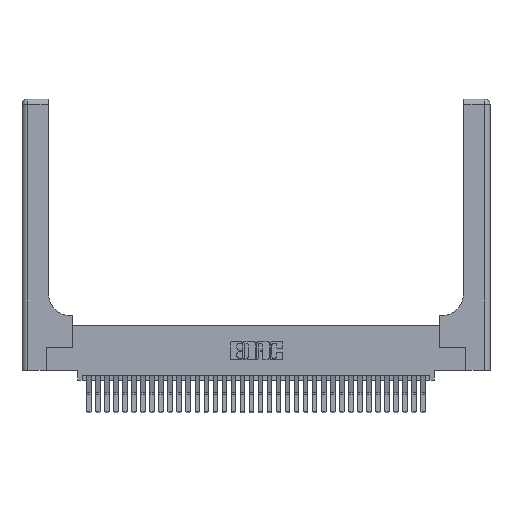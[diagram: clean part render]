
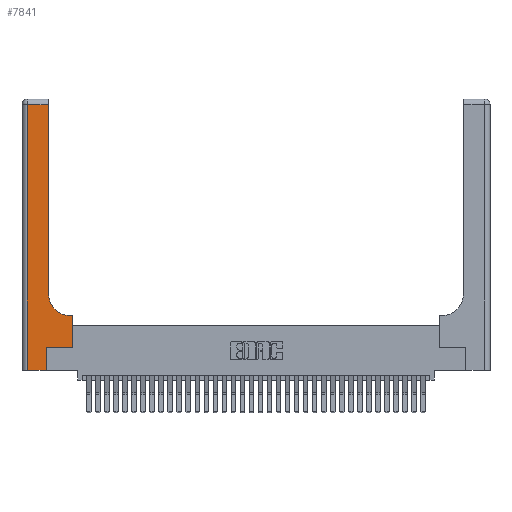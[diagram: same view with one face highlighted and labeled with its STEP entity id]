
A CAD part, top view. The second image highlights one B-rep face of the part: STEP entity #7841.
In plain terms, the highlighted planar face has unit normal (0, 0, 1).
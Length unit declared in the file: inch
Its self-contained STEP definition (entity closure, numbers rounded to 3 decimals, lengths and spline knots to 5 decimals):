
#426 = CARTESIAN_POINT ( 'NONE',  ( 0.269, 0.25, 0.37 ) ) ;
#1033 = VECTOR ( 'NONE', #4936, 39.37008 ) ;
#1945 = CARTESIAN_POINT ( 'NONE',  ( 0.269, 0., 0.37 ) ) ;
#1980 = VERTEX_POINT ( 'NONE', #25222 ) ;
#2105 = CARTESIAN_POINT ( 'NONE',  ( 0.5415, 0.6, 0.37 ) ) ;
#3399 = DIRECTION ( 'NONE',  ( -1., 0., 0. ) ) ;
#4581 = LINE ( 'NONE', #19040, #26658 ) ;
#4936 = DIRECTION ( 'NONE',  ( -1., 0., 0. ) ) ;
#5378 = CIRCLE ( 'NONE', #33731, 0.25 ) ;
#5398 = CARTESIAN_POINT ( 'NONE',  ( 0.5585, 0.6, 0.37 ) ) ;
#6071 = EDGE_CURVE ( 'NONE', #14214, #15749, #16802, .T. ) ;
#6264 = DIRECTION ( 'NONE',  ( 1., 0., 0. ) ) ;
#7271 = AXIS2_PLACEMENT_3D ( 'NONE', #10672, #13492, #32707 ) ;
#7841 = ADVANCED_FACE ( 'NONE', ( #27554 ), #27189, .F. ) ;
#8028 = ORIENTED_EDGE ( 'NONE', *, *, #30906, .T. ) ;
#8592 = VECTOR ( 'NONE', #35034, 39.37008 ) ;
#8611 = LINE ( 'NONE', #20057, #23381 ) ;
#8677 = EDGE_CURVE ( 'NONE', #21150, #14214, #9319, .T. ) ;
#9066 = CARTESIAN_POINT ( 'NONE',  ( 0., 0., 0.37 ) ) ;
#9319 = LINE ( 'NONE', #29836, #1033 ) ;
#9471 = LINE ( 'NONE', #21410, #8592 ) ;
#9536 = LINE ( 'NONE', #21793, #16086 ) ;
#10106 = EDGE_LOOP ( 'NONE', ( #15019, #24937, #25781, #33918, #27497, #8028, #30090, #17206, #10663 ) ) ;
#10663 = ORIENTED_EDGE ( 'NONE', *, *, #26675, .T. ) ;
#10672 = CARTESIAN_POINT ( 'NONE',  ( 0., 3., 0.37 ) ) ;
#11138 = DIRECTION ( 'NONE',  ( 0., -1., 0. ) ) ;
#12805 = CARTESIAN_POINT ( 'NONE',  ( 0.2915, 0.85, 0.37 ) ) ;
#13264 = VERTEX_POINT ( 'NONE', #12805 ) ;
#13492 = DIRECTION ( 'NONE',  ( 0., 0., -1. ) ) ;
#13664 = EDGE_CURVE ( 'NONE', #20463, #32364, #8611, .T. ) ;
#13843 = DIRECTION ( 'NONE',  ( 0., 1., 0. ) ) ;
#14214 = VERTEX_POINT ( 'NONE', #27674 ) ;
#15019 = ORIENTED_EDGE ( 'NONE', *, *, #15459, .T. ) ;
#15459 = EDGE_CURVE ( 'NONE', #13264, #21150, #4581, .T. ) ;
#15749 = VERTEX_POINT ( 'NONE', #28512 ) ;
#16086 = VECTOR ( 'NONE', #27171, 39.37008 ) ;
#16357 = DIRECTION ( 'NONE',  ( 0., 0., -1. ) ) ;
#16802 = LINE ( 'NONE', #27669, #22389 ) ;
#17206 = ORIENTED_EDGE ( 'NONE', *, *, #13664, .T. ) ;
#17605 = LINE ( 'NONE', #9066, #18465 ) ;
#18465 = VECTOR ( 'NONE', #6264, 39.37008 ) ;
#19040 = CARTESIAN_POINT ( 'NONE',  ( 0.2915, 3., 0.37 ) ) ;
#19464 = VERTEX_POINT ( 'NONE', #426 ) ;
#20057 = CARTESIAN_POINT ( 'NONE',  ( 0.2915, 0.6, 0.37 ) ) ;
#20463 = VERTEX_POINT ( 'NONE', #5398 ) ;
#21150 = VERTEX_POINT ( 'NONE', #33483 ) ;
#21222 = LINE ( 'NONE', #30325, #35745 ) ;
#21410 = CARTESIAN_POINT ( 'NONE',  ( 0.269, 0.25, 0.37 ) ) ;
#21793 = CARTESIAN_POINT ( 'NONE',  ( 0.5585, 0.25, 0.37 ) ) ;
#21798 = DIRECTION ( 'NONE',  ( 0., 1., 0. ) ) ;
#22079 = EDGE_CURVE ( 'NONE', #1980, #20463, #9536, .T. ) ;
#22389 = VECTOR ( 'NONE', #11138, 39.37008 ) ;
#23381 = VECTOR ( 'NONE', #3399, 39.37008 ) ;
#24937 = ORIENTED_EDGE ( 'NONE', *, *, #8677, .T. ) ;
#25222 = CARTESIAN_POINT ( 'NONE',  ( 0.5585, 0.25, 0.37 ) ) ;
#25343 = EDGE_CURVE ( 'NONE', #15749, #31587, #17605, .T. ) ;
#25781 = ORIENTED_EDGE ( 'NONE', *, *, #6071, .T. ) ;
#26658 = VECTOR ( 'NONE', #21798, 39.37008 ) ;
#26675 = EDGE_CURVE ( 'NONE', #32364, #13264, #5378, .T. ) ;
#27171 = DIRECTION ( 'NONE',  ( 0., 1., 0. ) ) ;
#27189 = PLANE ( 'NONE',  #7271 ) ;
#27497 = ORIENTED_EDGE ( 'NONE', *, *, #33828, .T. ) ;
#27554 = FACE_OUTER_BOUND ( 'NONE', #10106, .T. ) ;
#27669 = CARTESIAN_POINT ( 'NONE',  ( 0.06, 3., 0.37 ) ) ;
#27674 = CARTESIAN_POINT ( 'NONE',  ( 0.06, 2.94, 0.37 ) ) ;
#28512 = CARTESIAN_POINT ( 'NONE',  ( 0.06, 0., 0.37 ) ) ;
#29836 = CARTESIAN_POINT ( 'NONE',  ( 0., 2.94, 0.37 ) ) ;
#30090 = ORIENTED_EDGE ( 'NONE', *, *, #22079, .T. ) ;
#30325 = CARTESIAN_POINT ( 'NONE',  ( 0.269, 0., 0.37 ) ) ;
#30906 = EDGE_CURVE ( 'NONE', #19464, #1980, #9471, .T. ) ;
#31587 = VERTEX_POINT ( 'NONE', #1945 ) ;
#32364 = VERTEX_POINT ( 'NONE', #2105 ) ;
#32707 = DIRECTION ( 'NONE',  ( -1., 0., 0. ) ) ;
#32770 = CARTESIAN_POINT ( 'NONE',  ( 0.5415, 0.85, 0.37 ) ) ;
#33483 = CARTESIAN_POINT ( 'NONE',  ( 0.2915, 2.94, 0.37 ) ) ;
#33731 = AXIS2_PLACEMENT_3D ( 'NONE', #32770, #16357, #35490 ) ;
#33828 = EDGE_CURVE ( 'NONE', #31587, #19464, #21222, .T. ) ;
#33918 = ORIENTED_EDGE ( 'NONE', *, *, #25343, .T. ) ;
#35034 = DIRECTION ( 'NONE',  ( 1., 0., 0. ) ) ;
#35490 = DIRECTION ( 'NONE',  ( 1., 0., 0. ) ) ;
#35745 = VECTOR ( 'NONE', #13843, 39.37008 ) ;
